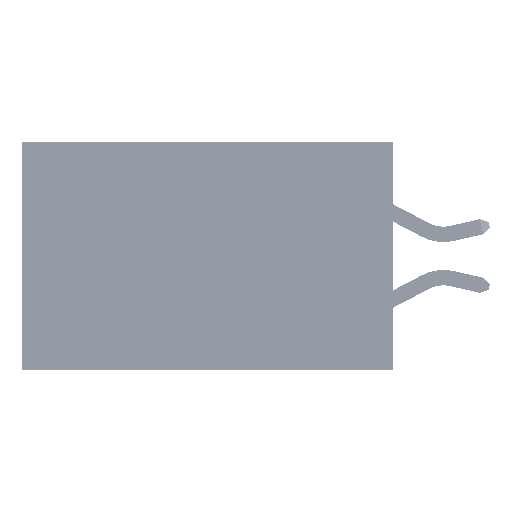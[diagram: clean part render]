
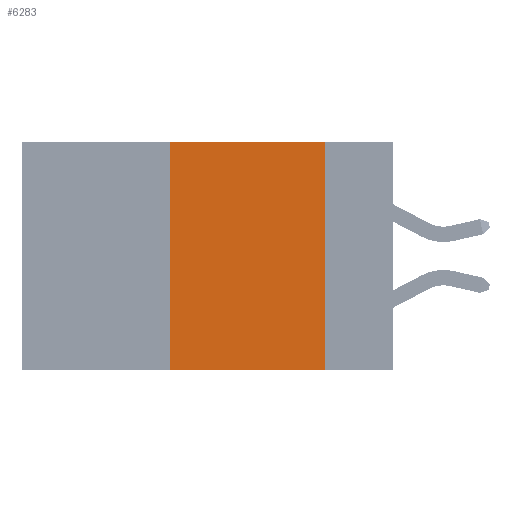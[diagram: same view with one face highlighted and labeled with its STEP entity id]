
A CAD part, left-side view. The second image highlights one B-rep face of the part: STEP entity #6283.
In plain terms, the highlighted planar face has unit normal (-1, 0, 0).
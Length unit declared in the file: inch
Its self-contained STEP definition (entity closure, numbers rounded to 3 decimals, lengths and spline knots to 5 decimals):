
#501 = CARTESIAN_POINT ( 'NONE',  ( 0., 0.11, -0.37 ) ) ;
#1951 = CARTESIAN_POINT ( 'NONE',  ( 0., 0.6, 0. ) ) ;
#3087 = CARTESIAN_POINT ( 'NONE',  ( 0., 0.36, 0. ) ) ;
#3301 = LINE ( 'NONE', #4715, #26933 ) ;
#4715 = CARTESIAN_POINT ( 'NONE',  ( 0., 0.6, -0.37 ) ) ;
#6283 = ADVANCED_FACE ( 'NONE', ( #40829 ), #45626, .F. ) ;
#10945 = ORIENTED_EDGE ( 'NONE', *, *, #20437, .T. ) ;
#12519 = LINE ( 'NONE', #40000, #31828 ) ;
#13757 = VECTOR ( 'NONE', #35260, 39.37008 ) ;
#14038 = AXIS2_PLACEMENT_3D ( 'NONE', #1951, #25583, #49763 ) ;
#14716 = EDGE_CURVE ( 'NONE', #15464, #46326, #29627, .T. ) ;
#15464 = VERTEX_POINT ( 'NONE', #41332 ) ;
#20437 = EDGE_CURVE ( 'NONE', #30877, #46326, #3301, .T. ) ;
#22096 = ORIENTED_EDGE ( 'NONE', *, *, #14716, .F. ) ;
#22478 = LINE ( 'NONE', #47302, #13757 ) ;
#24625 = VECTOR ( 'NONE', #37376, 39.37008 ) ;
#25583 = DIRECTION ( 'NONE',  ( 1., 0., 0. ) ) ;
#25704 = CARTESIAN_POINT ( 'NONE',  ( 0., 0.11, 0. ) ) ;
#25715 = ORIENTED_EDGE ( 'NONE', *, *, #26590, .F. ) ;
#26590 = EDGE_CURVE ( 'NONE', #27304, #15464, #12519, .T. ) ;
#26933 = VECTOR ( 'NONE', #32011, 39.37008 ) ;
#27304 = VERTEX_POINT ( 'NONE', #3087 ) ;
#29627 = LINE ( 'NONE', #25704, #24625 ) ;
#30288 = EDGE_LOOP ( 'NONE', ( #22096, #25715, #42895, #10945 ) ) ;
#30877 = VERTEX_POINT ( 'NONE', #33634 ) ;
#31828 = VECTOR ( 'NONE', #43851, 39.37008 ) ;
#32011 = DIRECTION ( 'NONE',  ( 0., -1., 0. ) ) ;
#33634 = CARTESIAN_POINT ( 'NONE',  ( 0., 0.36, -0.37 ) ) ;
#35260 = DIRECTION ( 'NONE',  ( 0., 0., 1. ) ) ;
#37376 = DIRECTION ( 'NONE',  ( 0., 0., -1. ) ) ;
#40000 = CARTESIAN_POINT ( 'NONE',  ( 0., 0.6, 0. ) ) ;
#40829 = FACE_OUTER_BOUND ( 'NONE', #30288, .T. ) ;
#41332 = CARTESIAN_POINT ( 'NONE',  ( 0., 0.11, 0. ) ) ;
#42895 = ORIENTED_EDGE ( 'NONE', *, *, #51476, .F. ) ;
#43851 = DIRECTION ( 'NONE',  ( 0., -1., 0. ) ) ;
#45626 = PLANE ( 'NONE',  #14038 ) ;
#46326 = VERTEX_POINT ( 'NONE', #501 ) ;
#47302 = CARTESIAN_POINT ( 'NONE',  ( 0., 0.36, 0. ) ) ;
#49763 = DIRECTION ( 'NONE',  ( 0., 0., -1. ) ) ;
#51476 = EDGE_CURVE ( 'NONE', #30877, #27304, #22478, .T. ) ;
